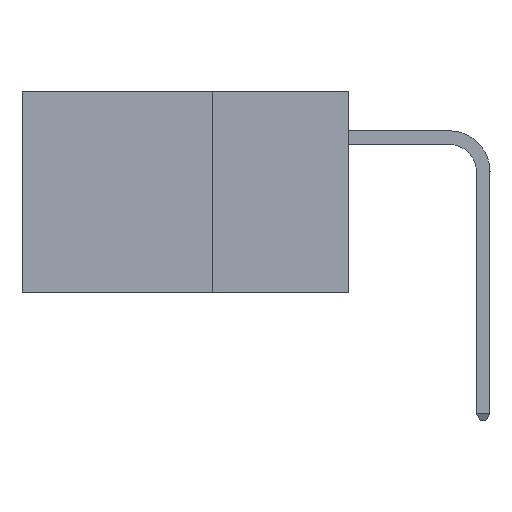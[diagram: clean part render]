
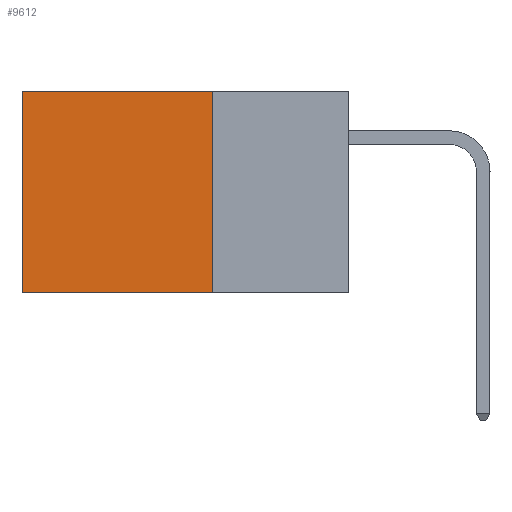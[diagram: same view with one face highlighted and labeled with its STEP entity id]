
A CAD part, left-side view. The second image highlights one B-rep face of the part: STEP entity #9612.
In plain terms, the highlighted planar face has unit normal (-1, 0, 0).
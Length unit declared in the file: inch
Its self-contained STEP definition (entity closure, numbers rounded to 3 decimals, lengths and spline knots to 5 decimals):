
#365 = EDGE_CURVE ( 'NONE', #5858, #2378, #4794, .T. ) ;
#552 = ORIENTED_EDGE ( 'NONE', *, *, #365, .F. ) ;
#629 = ORIENTED_EDGE ( 'NONE', *, *, #8132, .F. ) ;
#1126 = CARTESIAN_POINT ( 'NONE',  ( 0.2875, 0.6, 0. ) ) ;
#1251 = DIRECTION ( 'NONE',  ( 0., 0., -1. ) ) ;
#1495 = CARTESIAN_POINT ( 'NONE',  ( 0.2875, 0.25, 0. ) ) ;
#1550 = VECTOR ( 'NONE', #1251, 39.37008 ) ;
#1712 = LINE ( 'NONE', #6438, #8779 ) ;
#2070 = VECTOR ( 'NONE', #3984, 39.37008 ) ;
#2378 = VERTEX_POINT ( 'NONE', #5594 ) ;
#2471 = CARTESIAN_POINT ( 'NONE',  ( 0.2875, 0.25, 0. ) ) ;
#2778 = AXIS2_PLACEMENT_3D ( 'NONE', #9241, #4713, #9476 ) ;
#3167 = LINE ( 'NONE', #1126, #1550 ) ;
#3782 = FACE_OUTER_BOUND ( 'NONE', #4184, .T. ) ;
#3984 = DIRECTION ( 'NONE',  ( 0., 1., 0. ) ) ;
#4129 = VECTOR ( 'NONE', #4221, 39.37008 ) ;
#4184 = EDGE_LOOP ( 'NONE', ( #10735, #552, #629, #12061 ) ) ;
#4221 = DIRECTION ( 'NONE',  ( 0., 0., -1. ) ) ;
#4334 = VERTEX_POINT ( 'NONE', #2471 ) ;
#4420 = VERTEX_POINT ( 'NONE', #4525 ) ;
#4525 = CARTESIAN_POINT ( 'NONE',  ( 0.2875, 0.6, 0. ) ) ;
#4713 = DIRECTION ( 'NONE',  ( 1., 0., 0. ) ) ;
#4794 = LINE ( 'NONE', #4976, #2070 ) ;
#4976 = CARTESIAN_POINT ( 'NONE',  ( 0.2875, 0.25, -0.37 ) ) ;
#4977 = EDGE_CURVE ( 'NONE', #4420, #2378, #3167, .T. ) ;
#5277 = LINE ( 'NONE', #1495, #4129 ) ;
#5414 = PLANE ( 'NONE',  #2778 ) ;
#5594 = CARTESIAN_POINT ( 'NONE',  ( 0.2875, 0.6, -0.37 ) ) ;
#5726 = DIRECTION ( 'NONE',  ( 0., 1., 0. ) ) ;
#5858 = VERTEX_POINT ( 'NONE', #5935 ) ;
#5935 = CARTESIAN_POINT ( 'NONE',  ( 0.2875, 0.25, -0.37 ) ) ;
#6438 = CARTESIAN_POINT ( 'NONE',  ( 0.2875, 0.25, 0. ) ) ;
#8132 = EDGE_CURVE ( 'NONE', #4334, #5858, #5277, .T. ) ;
#8779 = VECTOR ( 'NONE', #5726, 39.37008 ) ;
#9241 = CARTESIAN_POINT ( 'NONE',  ( 0.2875, 0.25, 0. ) ) ;
#9476 = DIRECTION ( 'NONE',  ( 0., 0., -1. ) ) ;
#9612 = ADVANCED_FACE ( 'NONE', ( #3782 ), #5414, .F. ) ;
#10735 = ORIENTED_EDGE ( 'NONE', *, *, #4977, .T. ) ;
#12061 = ORIENTED_EDGE ( 'NONE', *, *, #12177, .T. ) ;
#12177 = EDGE_CURVE ( 'NONE', #4334, #4420, #1712, .T. ) ;
